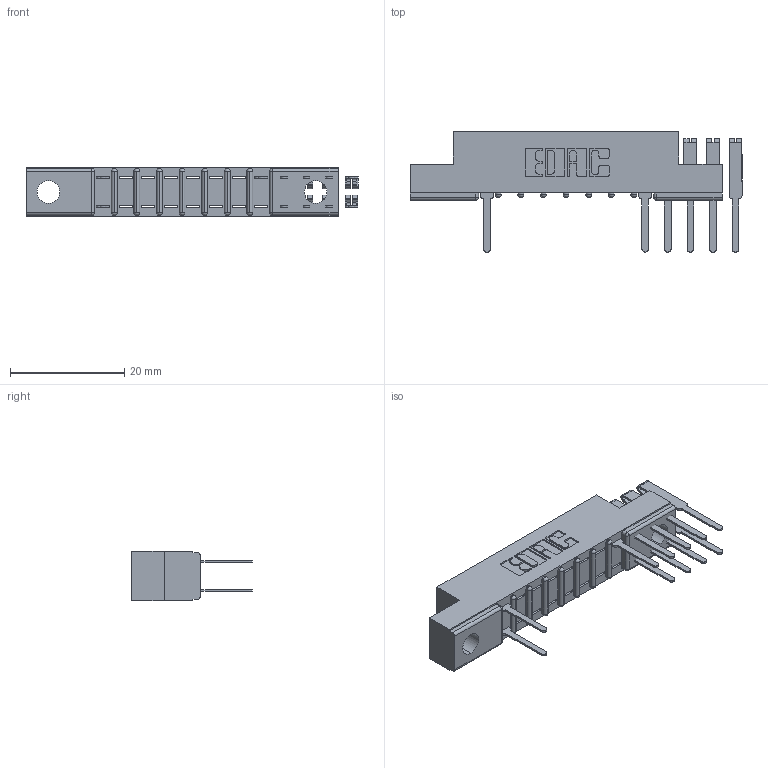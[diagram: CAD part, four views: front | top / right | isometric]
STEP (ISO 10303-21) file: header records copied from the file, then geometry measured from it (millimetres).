
FILE_DESCRIPTION (( 'STEP AP203' ), '1' );
FILE_NAME ('357-024-522-204.STEP', '2018-08-09T00:56:12', ( '' ), ( '' ), 'SwSTEP 2.0', 'SolidWorks 2016', '' );
FILE_SCHEMA (( 'CONFIG_CONTROL_DESIGN' ));
Length unit declared in the file: inch
Products named in the file (3): 307-290-001_522; 357-024-522-204; 307 Part_.156 Dia Mounting Holes
Assembly tree (12 placements, depth 2):
  357-024-522-204
    307 Part_.156 Dia Mounting Holes
    307-290-001_522  x11
Bounding box: 58.2 x 21.11 x 8.71 mm (x, y, z)
Volume: 3433.3 mm3; surface area: 4964.1 mm2
Topology: 12 solids, 12 shells, 697 faces, 1949 edges, 1258 vertices
Faces by surface type: plane 455, cylinder 224, sphere 18
Entity records: 11532 total; most frequent: CARTESIAN_POINT 1921, ORIENTED_EDGE 1902, DIRECTION 1883, EDGE_CURVE 951, VECTOR 723, LINE 723, VERTEX_POINT 618, AXIS2_PLACEMENT_3D 580
